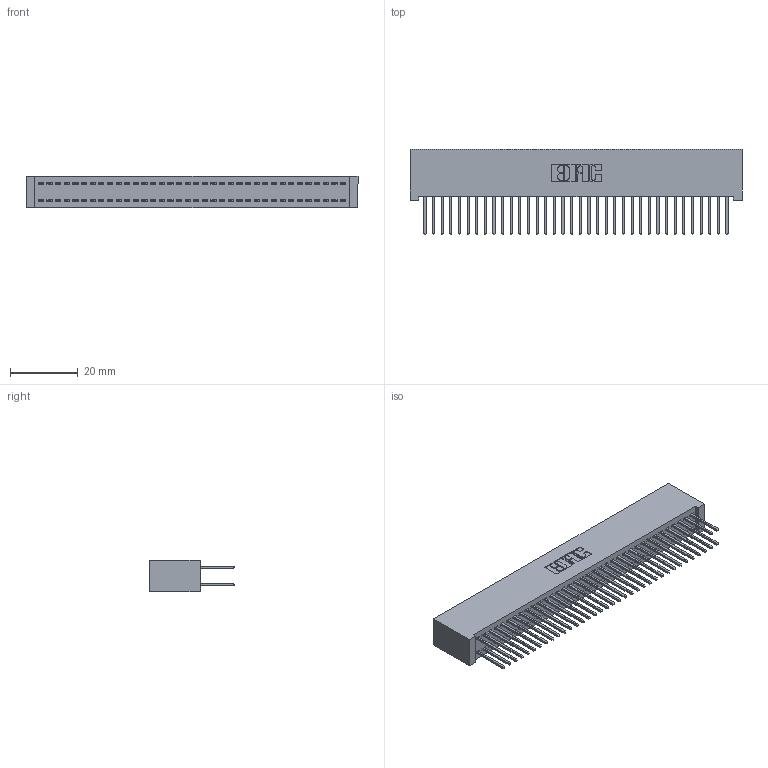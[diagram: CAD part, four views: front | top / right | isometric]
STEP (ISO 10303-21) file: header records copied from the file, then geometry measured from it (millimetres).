
FILE_DESCRIPTION (( 'STEP AP203' ), '1' );
FILE_NAME ('342-072-523-201.STEP', '2019-10-03T16:30:27', ( '' ), ( '' ), 'SwSTEP 2.0', 'SolidWorks 2016', '' );
FILE_SCHEMA (( 'CONFIG_CONTROL_DESIGN' ));
Length unit declared in the file: inch
Products named in the file (3): 342 Part_Lugless; 345-292-001_345-293-123; 342-072-523-201
Assembly tree (73 placements, depth 2):
  342-072-523-201
    342 Part_Lugless
    345-292-001_345-293-123  x72
Bounding box: 97.69 x 25.15 x 9.4 mm (x, y, z)
Volume: 9336 mm3; surface area: 16122.8 mm2
Topology: 73 solids, 73 shells, 3846 faces, 11435 edges, 7526 vertices
Faces by surface type: plane 2654, cylinder 1192
Entity records: 23545 total; most frequent: CARTESIAN_POINT 3906, ORIENTED_EDGE 3842, DIRECTION 3341, EDGE_CURVE 1921, LINE 1801, VECTOR 1801, VERTEX_POINT 1278, AXIS2_PLACEMENT_3D 770
